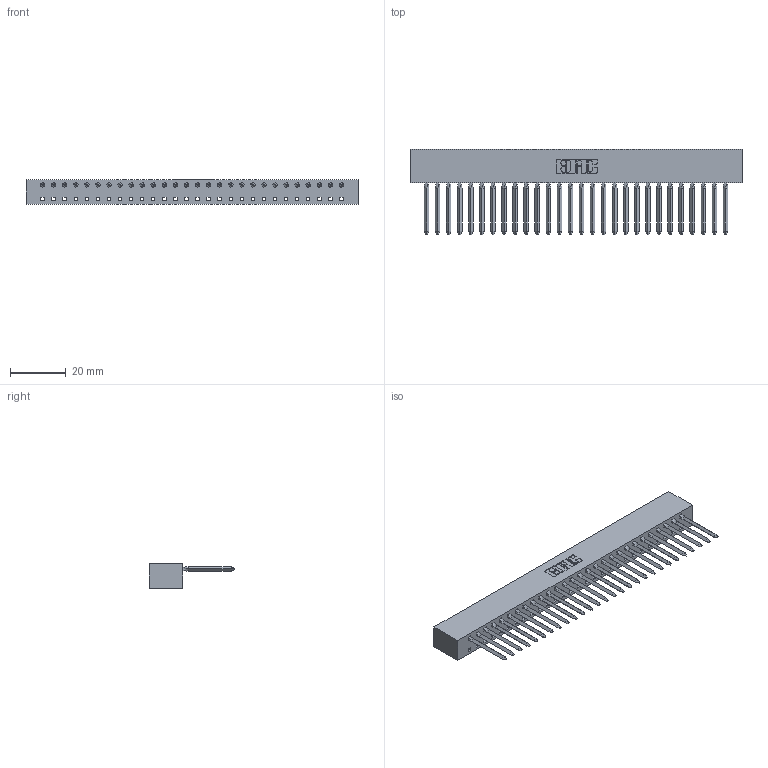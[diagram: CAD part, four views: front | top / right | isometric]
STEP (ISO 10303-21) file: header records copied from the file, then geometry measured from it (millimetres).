
FILE_DESCRIPTION (( 'STEP AP203' ), '1' );
FILE_NAME ('338-028-541-101.STEP', '2020-03-24T17:57:23', ( '' ), ( '' ), 'SwSTEP 2.0', 'SolidWorks 2016', '' );
FILE_SCHEMA (( 'CONFIG_CONTROL_DESIGN' ));
Length unit declared in the file: inch
Products named in the file (3): 338-028-541-101; 338-290-001_541; 338-210-001_338-210-028-001
Assembly tree (29 placements, depth 2):
  338-028-541-101
    338-210-001_338-210-028-001
    338-290-001_541  x28
Bounding box: 118.82 x 30.56 x 8.71 mm (x, y, z)
Volume: 8631.7 mm3; surface area: 14527.2 mm2
Topology: 29 solids, 29 shells, 2690 faces, 7423 edges, 4742 vertices
Faces by surface type: plane 1866, cylinder 712, bspline 112
Entity records: 54834 total; most frequent: CARTESIAN_POINT 11028, ORIENTED_EDGE 9284, DIRECTION 8653, EDGE_CURVE 4642, VECTOR 3471, LINE 3471, VERTEX_POINT 3014, AXIS2_PLACEMENT_3D 2591
